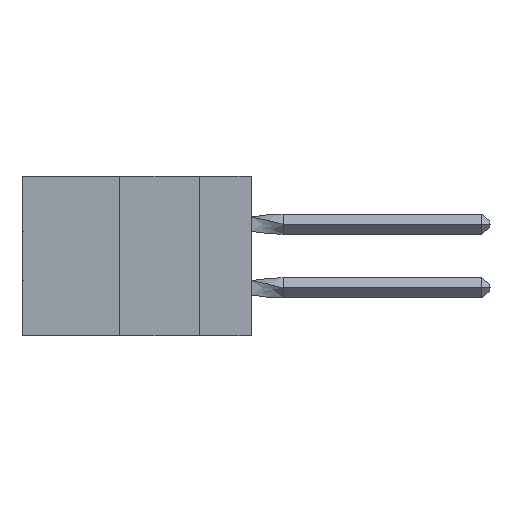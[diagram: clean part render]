
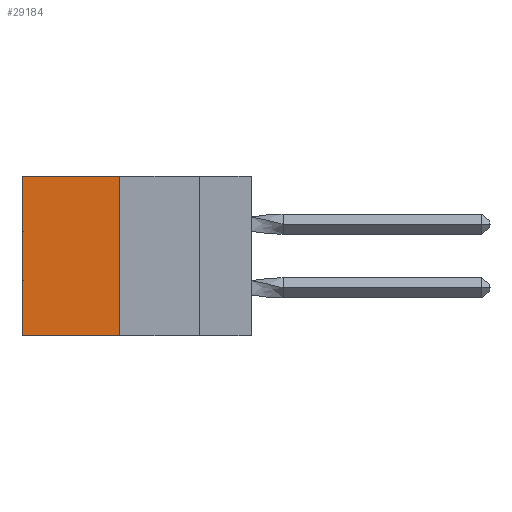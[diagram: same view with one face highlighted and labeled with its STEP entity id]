
A CAD part, left-side view. The second image highlights one B-rep face of the part: STEP entity #29184.
In plain terms, the highlighted planar face has unit normal (-1, 0, 0).
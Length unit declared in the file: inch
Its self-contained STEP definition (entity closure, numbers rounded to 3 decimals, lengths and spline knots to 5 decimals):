
#82 = LINE ( 'NONE', #4839, #31687 ) ;
#2469 = VECTOR ( 'NONE', #41245, 39.37008 ) ;
#4605 = CARTESIAN_POINT ( 'NONE',  ( 0.305, 0.72, 0. ) ) ;
#4839 = CARTESIAN_POINT ( 'NONE',  ( 0.305, 0.413, -0.5 ) ) ;
#5118 = AXIS2_PLACEMENT_3D ( 'NONE', #33264, #15046, #19301 ) ;
#5464 = DIRECTION ( 'NONE',  ( 0., 1., 0. ) ) ;
#6036 = EDGE_CURVE ( 'NONE', #45446, #20193, #23207, .T. ) ;
#7309 = VECTOR ( 'NONE', #46260, 39.37008 ) ;
#7912 = VERTEX_POINT ( 'NONE', #11536 ) ;
#8651 = VERTEX_POINT ( 'NONE', #37967 ) ;
#11536 = CARTESIAN_POINT ( 'NONE',  ( 0.305, 0.413, -0.5 ) ) ;
#11898 = PLANE ( 'NONE',  #5118 ) ;
#12612 = ORIENTED_EDGE ( 'NONE', *, *, #35319, .F. ) ;
#12812 = FACE_OUTER_BOUND ( 'NONE', #15940, .T. ) ;
#13419 = CARTESIAN_POINT ( 'NONE',  ( 0.305, 0.413, -0.5 ) ) ;
#15046 = DIRECTION ( 'NONE',  ( 1., 0., 0. ) ) ;
#15940 = EDGE_LOOP ( 'NONE', ( #16301, #17501, #12612, #28511 ) ) ;
#16301 = ORIENTED_EDGE ( 'NONE', *, *, #6036, .T. ) ;
#17041 = LINE ( 'NONE', #24740, #7309 ) ;
#17501 = ORIENTED_EDGE ( 'NONE', *, *, #42155, .F. ) ;
#19301 = DIRECTION ( 'NONE',  ( 0., 0., -1. ) ) ;
#20193 = VERTEX_POINT ( 'NONE', #37584 ) ;
#23207 = LINE ( 'NONE', #43825, #2469 ) ;
#24740 = CARTESIAN_POINT ( 'NONE',  ( 0.305, 0.413, 0. ) ) ;
#28511 = ORIENTED_EDGE ( 'NONE', *, *, #32783, .T. ) ;
#29184 = ADVANCED_FACE ( 'NONE', ( #12812 ), #11898, .F. ) ;
#31581 = DIRECTION ( 'NONE',  ( 0., 0., -1. ) ) ;
#31687 = VECTOR ( 'NONE', #5464, 39.37008 ) ;
#32783 = EDGE_CURVE ( 'NONE', #8651, #45446, #17041, .T. ) ;
#33264 = CARTESIAN_POINT ( 'NONE',  ( 0.305, 0.413, -0.5 ) ) ;
#35319 = EDGE_CURVE ( 'NONE', #8651, #7912, #39102, .T. ) ;
#36793 = VECTOR ( 'NONE', #31581, 39.37008 ) ;
#37584 = CARTESIAN_POINT ( 'NONE',  ( 0.305, 0.72, -0.5 ) ) ;
#37967 = CARTESIAN_POINT ( 'NONE',  ( 0.305, 0.413, 0. ) ) ;
#39102 = LINE ( 'NONE', #13419, #36793 ) ;
#41245 = DIRECTION ( 'NONE',  ( 0., 0., -1. ) ) ;
#42155 = EDGE_CURVE ( 'NONE', #7912, #20193, #82, .T. ) ;
#43825 = CARTESIAN_POINT ( 'NONE',  ( 0.305, 0.72, -0.5 ) ) ;
#45446 = VERTEX_POINT ( 'NONE', #4605 ) ;
#46260 = DIRECTION ( 'NONE',  ( 0., 1., 0. ) ) ;
